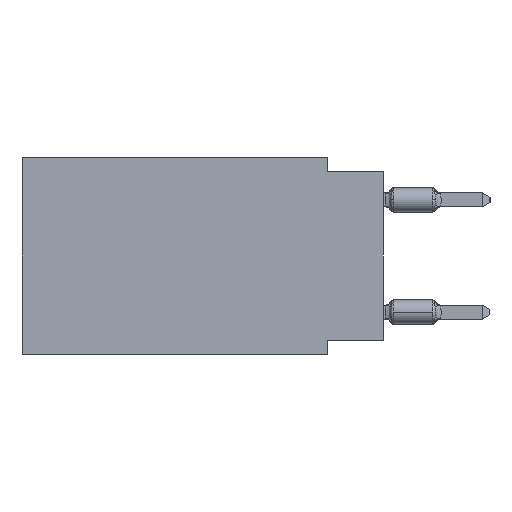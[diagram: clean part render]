
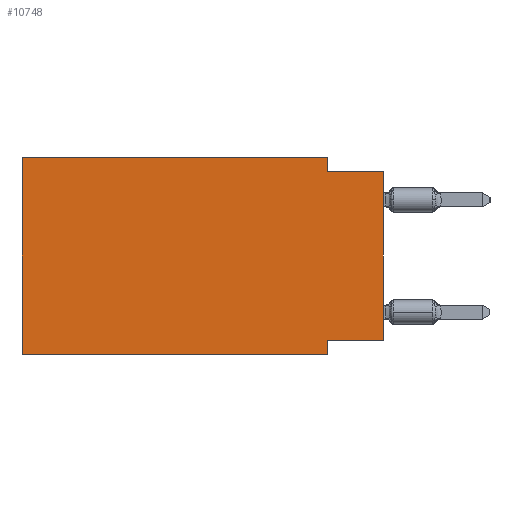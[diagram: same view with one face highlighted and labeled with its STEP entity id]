
A CAD part, left-side view. The second image highlights one B-rep face of the part: STEP entity #10748.
In plain terms, the highlighted planar face has unit normal (-1, 0, 0).
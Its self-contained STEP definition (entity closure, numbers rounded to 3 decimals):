
#29 = CARTESIAN_POINT ( 'NONE',  ( 0., 16.383, 0. ) ) ;
#795 = CARTESIAN_POINT ( 'NONE',  ( 0., 2.54, -0.635 ) ) ;
#954 = ORIENTED_EDGE ( 'NONE', *, *, #13794, .T. ) ;
#1524 = EDGE_CURVE ( 'NONE', #28388, #22141, #32614, .T. ) ;
#1689 = EDGE_CURVE ( 'NONE', #19583, #36309, #21874, .T. ) ;
#2296 = VERTEX_POINT ( 'NONE', #27013 ) ;
#2690 = VECTOR ( 'NONE', #35020, 1000. ) ;
#3339 = CARTESIAN_POINT ( 'NONE',  ( 0., 2.54, 0. ) ) ;
#4307 = VECTOR ( 'NONE', #10877, 1000. ) ;
#4375 = VERTEX_POINT ( 'NONE', #34076 ) ;
#4488 = DIRECTION ( 'NONE',  ( 0., 0., 1. ) ) ;
#4792 = CARTESIAN_POINT ( 'NONE',  ( 0., 16.383, 0. ) ) ;
#5174 = CARTESIAN_POINT ( 'NONE',  ( 0., 2.54, 0. ) ) ;
#5249 = ORIENTED_EDGE ( 'NONE', *, *, #38508, .F. ) ;
#5355 = CARTESIAN_POINT ( 'NONE',  ( 0., 2.54, -8.89 ) ) ;
#5699 = DIRECTION ( 'NONE',  ( 0., 0., 1. ) ) ;
#5855 = VECTOR ( 'NONE', #15016, 1000. ) ;
#5860 = ORIENTED_EDGE ( 'NONE', *, *, #1689, .F. ) ;
#6173 = VECTOR ( 'NONE', #8075, 1000. ) ;
#6294 = CARTESIAN_POINT ( 'NONE',  ( 0., 16.383, -8.89 ) ) ;
#6857 = CARTESIAN_POINT ( 'NONE',  ( 0., 16.383, 0. ) ) ;
#7326 = EDGE_LOOP ( 'NONE', ( #954, #5249, #32497, #25088, #29827, #31920, #8487, #5860 ) ) ;
#7886 = LINE ( 'NONE', #28770, #6173 ) ;
#8075 = DIRECTION ( 'NONE',  ( 0., -1., 0. ) ) ;
#8487 = ORIENTED_EDGE ( 'NONE', *, *, #32515, .F. ) ;
#9472 = EDGE_CURVE ( 'NONE', #18716, #2296, #7886, .T. ) ;
#10584 = FACE_OUTER_BOUND ( 'NONE', #7326, .T. ) ;
#10748 = ADVANCED_FACE ( 'NONE', ( #10584 ), #34393, .F. ) ;
#10877 = DIRECTION ( 'NONE',  ( 0., 1., 0. ) ) ;
#13129 = DIRECTION ( 'NONE',  ( 1., 0., 0. ) ) ;
#13794 = EDGE_CURVE ( 'NONE', #19583, #4375, #18005, .T. ) ;
#14825 = LINE ( 'NONE', #29673, #5855 ) ;
#15016 = DIRECTION ( 'NONE',  ( 0., -1., 0. ) ) ;
#15681 = VECTOR ( 'NONE', #4488, 1000. ) ;
#16053 = CARTESIAN_POINT ( 'NONE',  ( 0., 16.383, 0. ) ) ;
#16888 = LINE ( 'NONE', #5355, #2690 ) ;
#17131 = EDGE_CURVE ( 'NONE', #32598, #28388, #24634, .T. ) ;
#18005 = LINE ( 'NONE', #34994, #30156 ) ;
#18716 = VERTEX_POINT ( 'NONE', #6294 ) ;
#19583 = VERTEX_POINT ( 'NONE', #32367 ) ;
#21819 = AXIS2_PLACEMENT_3D ( 'NONE', #16053, #13129, #37311 ) ;
#21874 = LINE ( 'NONE', #33771, #4307 ) ;
#22141 = VERTEX_POINT ( 'NONE', #795 ) ;
#22217 = EDGE_CURVE ( 'NONE', #18716, #32598, #26772, .T. ) ;
#24634 = LINE ( 'NONE', #6857, #31248 ) ;
#25088 = ORIENTED_EDGE ( 'NONE', *, *, #17131, .F. ) ;
#26656 = DIRECTION ( 'NONE',  ( 0., -1., 0. ) ) ;
#26772 = LINE ( 'NONE', #29, #15681 ) ;
#27013 = CARTESIAN_POINT ( 'NONE',  ( 0., 2.54, -8.89 ) ) ;
#28388 = VERTEX_POINT ( 'NONE', #5174 ) ;
#28770 = CARTESIAN_POINT ( 'NONE',  ( 0., 16.383, -8.89 ) ) ;
#29673 = CARTESIAN_POINT ( 'NONE',  ( 0., 0., -0.635 ) ) ;
#29827 = ORIENTED_EDGE ( 'NONE', *, *, #22217, .F. ) ;
#30156 = VECTOR ( 'NONE', #5699, 1000. ) ;
#30272 = DIRECTION ( 'NONE',  ( 0., 0., -1. ) ) ;
#31248 = VECTOR ( 'NONE', #26656, 1000. ) ;
#31920 = ORIENTED_EDGE ( 'NONE', *, *, #9472, .T. ) ;
#32367 = CARTESIAN_POINT ( 'NONE',  ( 0., 0., -8.255 ) ) ;
#32497 = ORIENTED_EDGE ( 'NONE', *, *, #1524, .F. ) ;
#32515 = EDGE_CURVE ( 'NONE', #36309, #2296, #16888, .T. ) ;
#32598 = VERTEX_POINT ( 'NONE', #4792 ) ;
#32614 = LINE ( 'NONE', #3339, #34238 ) ;
#33771 = CARTESIAN_POINT ( 'NONE',  ( 0., 0., -8.255 ) ) ;
#34076 = CARTESIAN_POINT ( 'NONE',  ( 0., 0., -0.635 ) ) ;
#34238 = VECTOR ( 'NONE', #30272, 1000. ) ;
#34393 = PLANE ( 'NONE',  #21819 ) ;
#34994 = CARTESIAN_POINT ( 'NONE',  ( 0., 0., 0. ) ) ;
#35020 = DIRECTION ( 'NONE',  ( 0., 0., -1. ) ) ;
#35027 = CARTESIAN_POINT ( 'NONE',  ( 0., 2.54, -8.255 ) ) ;
#36309 = VERTEX_POINT ( 'NONE', #35027 ) ;
#37311 = DIRECTION ( 'NONE',  ( 0., 0., -1. ) ) ;
#38508 = EDGE_CURVE ( 'NONE', #22141, #4375, #14825, .T. ) ;
